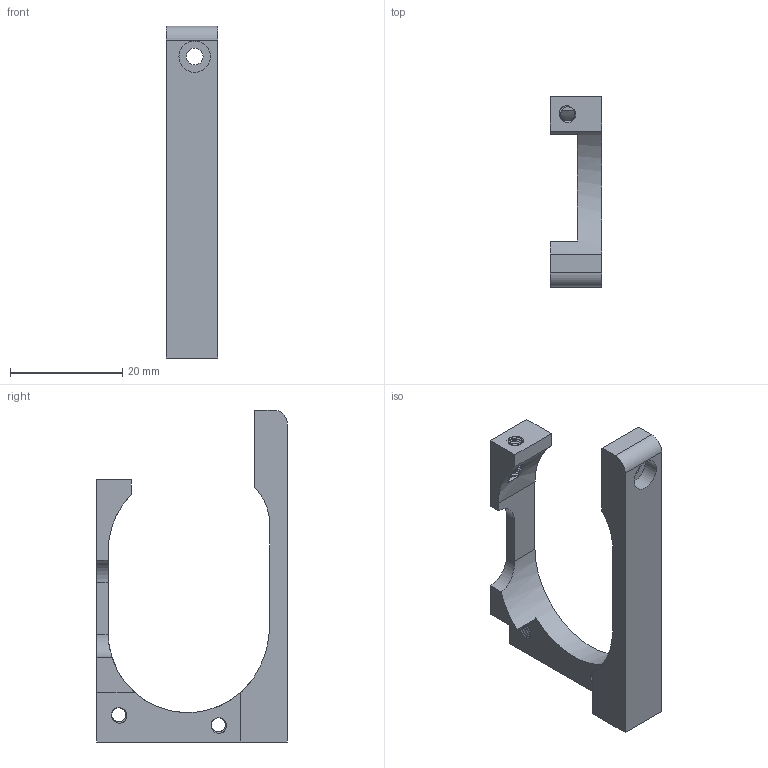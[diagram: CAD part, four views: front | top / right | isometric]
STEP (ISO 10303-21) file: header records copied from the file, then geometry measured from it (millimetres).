
FILE_DESCRIPTION(/* description */ (''),/* implementation_level */ '2;1');
FILE_NAME(/* name */ 'Left Trigger Guard.step',/* time_stamp */ '2024-01-16T15:55:44-05:00',/* author */ (''),/* organization */ (''),/* preprocessor_version */ 'ST-DEVELOPER v20',/* originating_system */ 'Autodesk Translation Framework v12.14.0.127',/* authorisation */ '');
FILE_SCHEMA (('AUTOMOTIVE_DESIGN { 1 0 10303 214 3 1 1 }'));
Length unit declared in the file: inch
Products named in the file (1): Left Trigger Guard
Bounding box: 9.22 x 34.06 x 59.26 mm (x, y, z)
Volume: 4262.3 mm3; surface area: 3570 mm2
Topology: 1 solids, 1 shells, 127 faces, 375 edges, 250 vertices
Faces by surface type: cylinder 87, bspline 21, plane 19
Full cylindrical faces by diameter (mm): 2.529 x16, 3 x1, 3.086 x12, 5.6 x1
Entity records: 8483 total; most frequent: CARTESIAN_POINT 5529, ORIENTED_EDGE 750, DIRECTION 384, EDGE_CURVE 375, VERTEX_POINT 250, B_SPLINE_CURVE_WITH_KNOTS 236, AXIS2_PLACEMENT_3D 138, EDGE_LOOP 137
